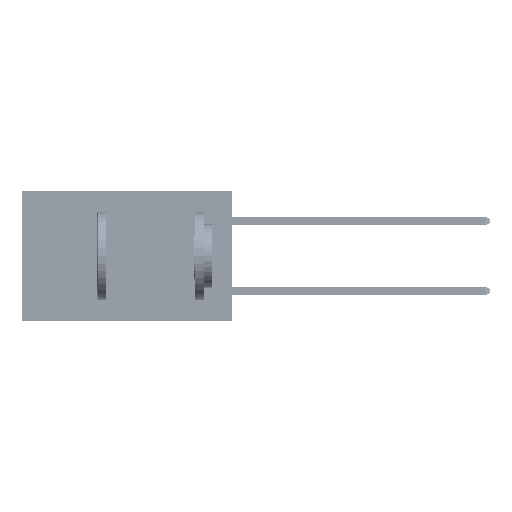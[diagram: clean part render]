
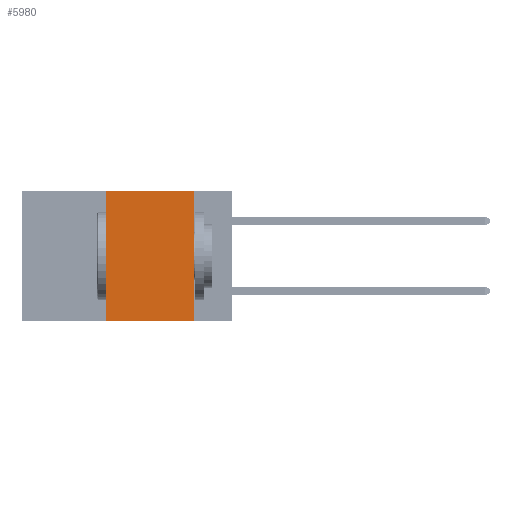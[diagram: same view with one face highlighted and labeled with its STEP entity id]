
A CAD part, left-side view. The second image highlights one B-rep face of the part: STEP entity #5980.
In plain terms, the highlighted planar face has unit normal (-1, 0, 0).
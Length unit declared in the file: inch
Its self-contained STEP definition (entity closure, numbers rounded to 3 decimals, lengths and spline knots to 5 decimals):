
#64 = CARTESIAN_POINT ( 'NONE',  ( 0., 0.11, 0. ) ) ;
#1236 = VERTEX_POINT ( 'NONE', #27596 ) ;
#1437 = CARTESIAN_POINT ( 'NONE',  ( 0., 0.11, -0.37 ) ) ;
#2617 = DIRECTION ( 'NONE',  ( 0., 0., -1. ) ) ;
#4341 = ORIENTED_EDGE ( 'NONE', *, *, #20792, .T. ) ;
#5980 = ADVANCED_FACE ( 'NONE', ( #15025 ), #28891, .F. ) ;
#6583 = CARTESIAN_POINT ( 'NONE',  ( 0., 0.11, 0. ) ) ;
#7806 = CARTESIAN_POINT ( 'NONE',  ( 0., 0.36, 0. ) ) ;
#9926 = DIRECTION ( 'NONE',  ( 0., 0., -1. ) ) ;
#14022 = DIRECTION ( 'NONE',  ( 1., 0., 0. ) ) ;
#14071 = LINE ( 'NONE', #41205, #30558 ) ;
#15025 = FACE_OUTER_BOUND ( 'NONE', #33246, .T. ) ;
#18258 = DIRECTION ( 'NONE',  ( 0., -1., 0. ) ) ;
#18594 = ORIENTED_EDGE ( 'NONE', *, *, #25025, .F. ) ;
#20466 = LINE ( 'NONE', #48293, #24576 ) ;
#20792 = EDGE_CURVE ( 'NONE', #1236, #41650, #31086, .T. ) ;
#22562 = EDGE_CURVE ( 'NONE', #47145, #37282, #14071, .T. ) ;
#24576 = VECTOR ( 'NONE', #32837, 39.37008 ) ;
#25025 = EDGE_CURVE ( 'NONE', #1236, #47145, #20466, .T. ) ;
#27596 = CARTESIAN_POINT ( 'NONE',  ( 0., 0.36, -0.37 ) ) ;
#28891 = PLANE ( 'NONE',  #43480 ) ;
#30558 = VECTOR ( 'NONE', #18258, 39.37008 ) ;
#31086 = LINE ( 'NONE', #44271, #33450 ) ;
#32837 = DIRECTION ( 'NONE',  ( 0., 0., 1. ) ) ;
#33246 = EDGE_LOOP ( 'NONE', ( #47971, #43434, #18594, #4341 ) ) ;
#33450 = VECTOR ( 'NONE', #44767, 39.37008 ) ;
#37282 = VERTEX_POINT ( 'NONE', #64 ) ;
#41152 = EDGE_CURVE ( 'NONE', #37282, #41650, #46580, .T. ) ;
#41205 = CARTESIAN_POINT ( 'NONE',  ( 0., 0.6, 0. ) ) ;
#41650 = VERTEX_POINT ( 'NONE', #1437 ) ;
#43069 = VECTOR ( 'NONE', #2617, 39.37008 ) ;
#43434 = ORIENTED_EDGE ( 'NONE', *, *, #22562, .F. ) ;
#43480 = AXIS2_PLACEMENT_3D ( 'NONE', #47651, #14022, #9926 ) ;
#44271 = CARTESIAN_POINT ( 'NONE',  ( 0., 0.6, -0.37 ) ) ;
#44767 = DIRECTION ( 'NONE',  ( 0., -1., 0. ) ) ;
#46580 = LINE ( 'NONE', #6583, #43069 ) ;
#47145 = VERTEX_POINT ( 'NONE', #7806 ) ;
#47651 = CARTESIAN_POINT ( 'NONE',  ( 0., 0.6, 0. ) ) ;
#47971 = ORIENTED_EDGE ( 'NONE', *, *, #41152, .F. ) ;
#48293 = CARTESIAN_POINT ( 'NONE',  ( 0., 0.36, 0. ) ) ;
